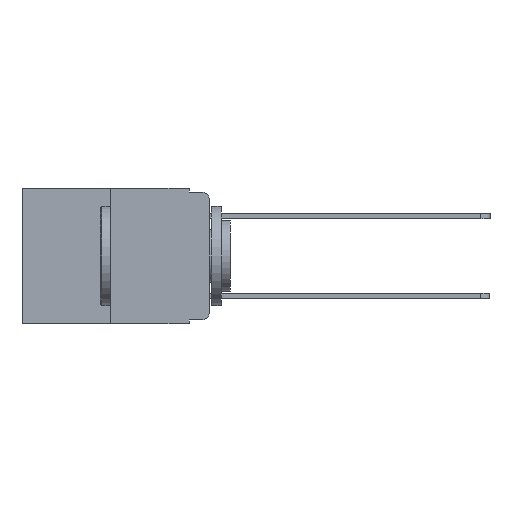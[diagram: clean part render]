
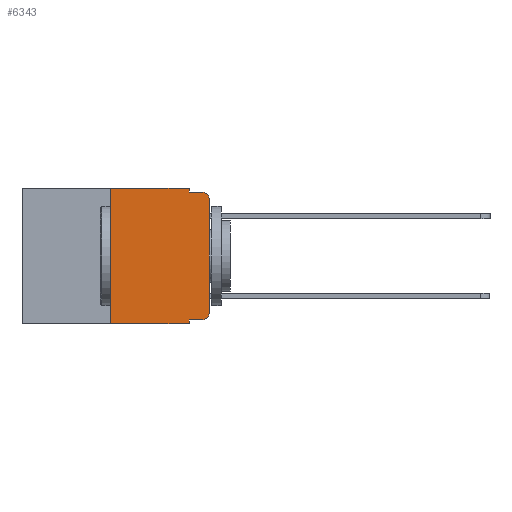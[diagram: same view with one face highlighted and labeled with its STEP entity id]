
A CAD part, left-side view. The second image highlights one B-rep face of the part: STEP entity #6343.
In plain terms, the highlighted planar face has unit normal (-1, 0, 0).
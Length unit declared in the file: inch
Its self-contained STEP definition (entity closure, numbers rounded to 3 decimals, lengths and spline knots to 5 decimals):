
#348 = CIRCLE ( 'NONE', #20000, 0.02 ) ;
#511 = CARTESIAN_POINT ( 'NONE',  ( 0., 0., -0.313 ) ) ;
#753 = FACE_OUTER_BOUND ( 'NONE', #13428, .T. ) ;
#1201 = CARTESIAN_POINT ( 'NONE',  ( 0., 0., -0.03 ) ) ;
#1612 = AXIS2_PLACEMENT_3D ( 'NONE', #3973, #19529, #9271 ) ;
#1731 = LINE ( 'NONE', #17502, #19633 ) ;
#2131 = CARTESIAN_POINT ( 'NONE',  ( 0., 0.051, 0. ) ) ;
#2358 = VERTEX_POINT ( 'NONE', #511 ) ;
#2465 = AXIS2_PLACEMENT_3D ( 'NONE', #8039, #20035, #9835 ) ;
#2737 = EDGE_CURVE ( 'NONE', #12713, #8968, #348, .T. ) ;
#3140 = CARTESIAN_POINT ( 'NONE',  ( 0., 0.473, -0.343 ) ) ;
#3973 = CARTESIAN_POINT ( 'NONE',  ( 0., 0.473, 0. ) ) ;
#4060 = DIRECTION ( 'NONE',  ( -1., 0., 0. ) ) ;
#4069 = EDGE_CURVE ( 'NONE', #2358, #12713, #13792, .T. ) ;
#4086 = CARTESIAN_POINT ( 'NONE',  ( 0., 0.02, -0.03 ) ) ;
#4566 = VERTEX_POINT ( 'NONE', #20281 ) ;
#4959 = VERTEX_POINT ( 'NONE', #22290 ) ;
#5357 = DIRECTION ( 'NONE',  ( 0., -1., 0. ) ) ;
#6063 = LINE ( 'NONE', #16624, #12687 ) ;
#6334 = VERTEX_POINT ( 'NONE', #2131 ) ;
#6343 = ADVANCED_FACE ( 'NONE', ( #753 ), #11002, .F. ) ;
#6846 = CARTESIAN_POINT ( 'NONE',  ( 0., 0.051, -0.01 ) ) ;
#7308 = ORIENTED_EDGE ( 'NONE', *, *, #8111, .F. ) ;
#8039 = CARTESIAN_POINT ( 'NONE',  ( 0., 0.02, -0.313 ) ) ;
#8111 = EDGE_CURVE ( 'NONE', #13866, #4959, #1731, .T. ) ;
#8700 = CARTESIAN_POINT ( 'NONE',  ( 0., 0.25, 0. ) ) ;
#8795 = ORIENTED_EDGE ( 'NONE', *, *, #10341, .F. ) ;
#8827 = CARTESIAN_POINT ( 'NONE',  ( 0., 0.473, 0. ) ) ;
#8968 = VERTEX_POINT ( 'NONE', #18206 ) ;
#9120 = VECTOR ( 'NONE', #10520, 39.37008 ) ;
#9242 = ORIENTED_EDGE ( 'NONE', *, *, #16975, .T. ) ;
#9271 = DIRECTION ( 'NONE',  ( 0., 0., -1. ) ) ;
#9382 = DIRECTION ( 'NONE',  ( 0., -1., 0. ) ) ;
#9573 = ORIENTED_EDGE ( 'NONE', *, *, #2737, .T. ) ;
#9835 = DIRECTION ( 'NONE',  ( 0., 0., -1. ) ) ;
#10022 = DIRECTION ( 'NONE',  ( 0., -1., 0. ) ) ;
#10341 = EDGE_CURVE ( 'NONE', #4566, #13990, #6063, .T. ) ;
#10415 = CARTESIAN_POINT ( 'NONE',  ( 0., 0.02, -0.333 ) ) ;
#10520 = DIRECTION ( 'NONE',  ( 0., 0., 1. ) ) ;
#10992 = VECTOR ( 'NONE', #9382, 39.37008 ) ;
#11002 = PLANE ( 'NONE',  #1612 ) ;
#11251 = EDGE_CURVE ( 'NONE', #18908, #2358, #16631, .T. ) ;
#12263 = EDGE_CURVE ( 'NONE', #6334, #15716, #20496, .T. ) ;
#12687 = VECTOR ( 'NONE', #21595, 39.37008 ) ;
#12713 = VERTEX_POINT ( 'NONE', #1201 ) ;
#12757 = EDGE_CURVE ( 'NONE', #4566, #4959, #14971, .T. ) ;
#13325 = ORIENTED_EDGE ( 'NONE', *, *, #19122, .F. ) ;
#13328 = ORIENTED_EDGE ( 'NONE', *, *, #12263, .F. ) ;
#13428 = EDGE_LOOP ( 'NONE', ( #17346, #9573, #13325, #13328, #18656, #8795, #15274, #7308, #9242, #16310 ) ) ;
#13537 = VECTOR ( 'NONE', #10022, 39.37008 ) ;
#13685 = DIRECTION ( 'NONE',  ( 0., -1., 0. ) ) ;
#13792 = LINE ( 'NONE', #16879, #9120 ) ;
#13866 = VERTEX_POINT ( 'NONE', #15337 ) ;
#13990 = VERTEX_POINT ( 'NONE', #8700 ) ;
#14079 = LINE ( 'NONE', #21841, #13537 ) ;
#14160 = DIRECTION ( 'NONE',  ( 0., 0., -1. ) ) ;
#14231 = VECTOR ( 'NONE', #5357, 39.37008 ) ;
#14971 = LINE ( 'NONE', #3140, #15517 ) ;
#15274 = ORIENTED_EDGE ( 'NONE', *, *, #12757, .T. ) ;
#15337 = CARTESIAN_POINT ( 'NONE',  ( 0., 0.051, -0.333 ) ) ;
#15385 = DIRECTION ( 'NONE',  ( 0., 0., -1. ) ) ;
#15517 = VECTOR ( 'NONE', #13685, 39.37008 ) ;
#15716 = VERTEX_POINT ( 'NONE', #6846 ) ;
#15905 = DIRECTION ( 'NONE',  ( 0., 0., -1. ) ) ;
#16115 = LINE ( 'NONE', #16295, #10992 ) ;
#16295 = CARTESIAN_POINT ( 'NONE',  ( 0., 0.051, -0.01 ) ) ;
#16310 = ORIENTED_EDGE ( 'NONE', *, *, #11251, .T. ) ;
#16624 = CARTESIAN_POINT ( 'NONE',  ( 0., 0.25, 0. ) ) ;
#16631 = CIRCLE ( 'NONE', #2465, 0.02 ) ;
#16879 = CARTESIAN_POINT ( 'NONE',  ( 0., 0., 0. ) ) ;
#16975 = EDGE_CURVE ( 'NONE', #13866, #18908, #14079, .T. ) ;
#17346 = ORIENTED_EDGE ( 'NONE', *, *, #4069, .T. ) ;
#17502 = CARTESIAN_POINT ( 'NONE',  ( 0., 0.051, 0. ) ) ;
#17536 = CARTESIAN_POINT ( 'NONE',  ( 0., 0.051, 0. ) ) ;
#18206 = CARTESIAN_POINT ( 'NONE',  ( 0., 0.02, -0.01 ) ) ;
#18656 = ORIENTED_EDGE ( 'NONE', *, *, #19820, .F. ) ;
#18908 = VERTEX_POINT ( 'NONE', #10415 ) ;
#19122 = EDGE_CURVE ( 'NONE', #15716, #8968, #16115, .T. ) ;
#19202 = LINE ( 'NONE', #8827, #14231 ) ;
#19529 = DIRECTION ( 'NONE',  ( 1., 0., 0. ) ) ;
#19633 = VECTOR ( 'NONE', #15905, 39.37008 ) ;
#19820 = EDGE_CURVE ( 'NONE', #13990, #6334, #19202, .T. ) ;
#19970 = VECTOR ( 'NONE', #14160, 39.37008 ) ;
#20000 = AXIS2_PLACEMENT_3D ( 'NONE', #4086, #4060, #15385 ) ;
#20035 = DIRECTION ( 'NONE',  ( -1., 0., 0. ) ) ;
#20281 = CARTESIAN_POINT ( 'NONE',  ( 0., 0.25, -0.343 ) ) ;
#20496 = LINE ( 'NONE', #17536, #19970 ) ;
#21595 = DIRECTION ( 'NONE',  ( 0., 0., 1. ) ) ;
#21841 = CARTESIAN_POINT ( 'NONE',  ( 0., 0.051, -0.333 ) ) ;
#22290 = CARTESIAN_POINT ( 'NONE',  ( 0., 0.051, -0.343 ) ) ;
